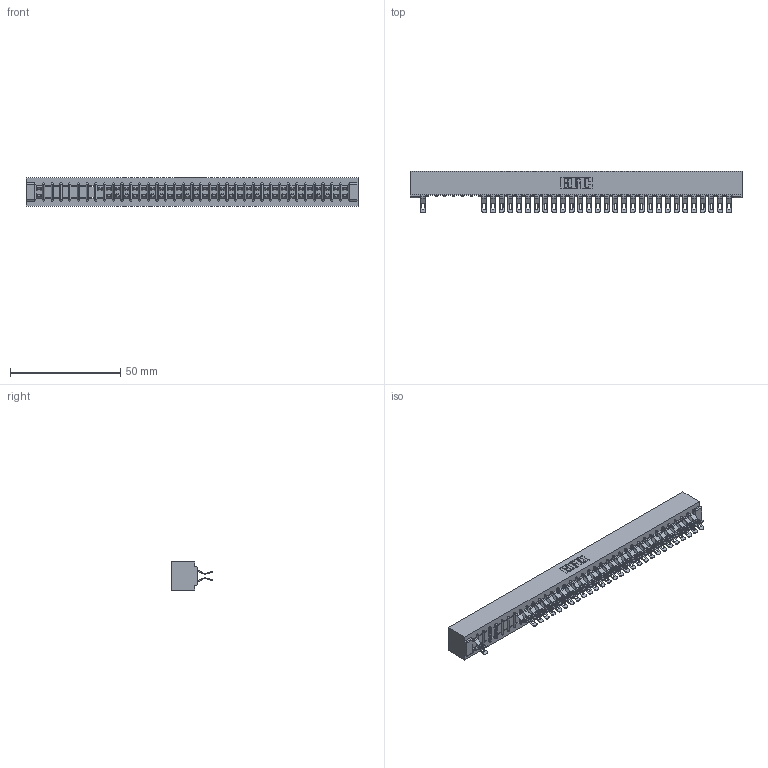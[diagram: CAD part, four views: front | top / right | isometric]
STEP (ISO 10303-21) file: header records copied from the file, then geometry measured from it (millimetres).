
FILE_DESCRIPTION (( 'STEP AP203' ), '1' );
FILE_NAME ('307-072-555-201.STEP', '2018-08-06T15:34:23', ( '' ), ( '' ), 'SwSTEP 2.0', 'SolidWorks 2016', '' );
FILE_SCHEMA (( 'CONFIG_CONTROL_DESIGN' ));
Length unit declared in the file: inch
Products named in the file (3): 307 Part_No Mounting Lugs; 307-290-001_555; 307-072-555-201
Assembly tree (60 placements, depth 2):
  307-072-555-201
    307 Part_No Mounting Lugs
    307-290-001_555  x59
Bounding box: 150.52 x 18.75 x 12.7 mm (x, y, z)
Volume: 16518.6 mm3; surface area: 20275.6 mm2
Topology: 60 solids, 60 shells, 3876 faces, 11394 edges, 7416 vertices
Faces by surface type: plane 2150, cylinder 1652, sphere 74
Entity records: 32597 total; most frequent: CARTESIAN_POINT 5391, ORIENTED_EDGE 5356, DIRECTION 5276, EDGE_CURVE 2678, LINE 2042, VECTOR 2042, VERTEX_POINT 1732, AXIS2_PLACEMENT_3D 1617
